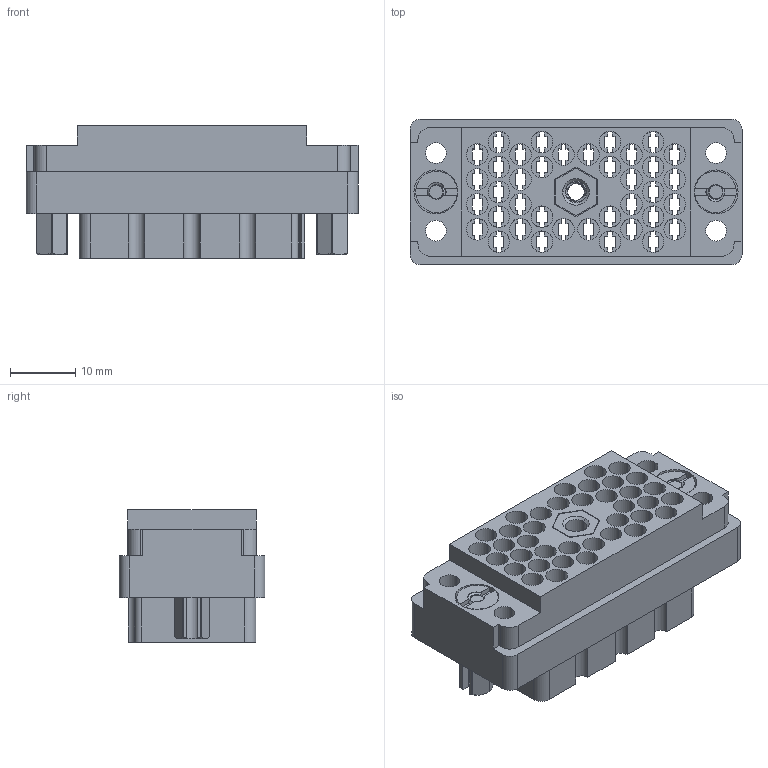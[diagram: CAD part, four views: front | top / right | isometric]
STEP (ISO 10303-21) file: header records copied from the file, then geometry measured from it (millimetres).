
FILE_DESCRIPTION (( 'STEP AP203' ), '1' );
FILE_NAME ('516-038-000-402.STEP', '2020-03-04T21:43:05', ( '' ), ( '' ), 'SwSTEP 2.0', 'SolidWorks 2016', '' );
FILE_SCHEMA (( 'CONFIG_CONTROL_DESIGN' ));
Length unit declared in the file: inch
Products named in the file (6): 516-252-035-100_516-252-035-100; 516-038-000-402; 516 Part Receptacle_038; 516-221-038-102_039; 516-252-021-102_038; 516-221-038-102_038
Assembly tree (6 placements, depth 2):
  516-038-000-402
    516 Part Receptacle_038
    516-252-021-102_038  x2
    516-221-038-102_038
    516-252-035-100_516-252-035-100
    516-221-038-102_039
Bounding box: 50.8 x 22.25 x 20.27 mm (x, y, z)
Volume: 11180 mm3; surface area: 15859.7 mm2
Topology: 6 solids, 6 shells, 1137 faces, 3288 edges, 2178 vertices
Faces by surface type: plane 695, cylinder 364, cone 44, bspline 34
Entity records: 43571 total; most frequent: CARTESIAN_POINT 13423, ORIENTED_EDGE 6388, DIRECTION 5995, EDGE_CURVE 3194, LINE 2139, VECTOR 2139, VERTEX_POINT 2118, AXIS2_PLACEMENT_3D 1928
